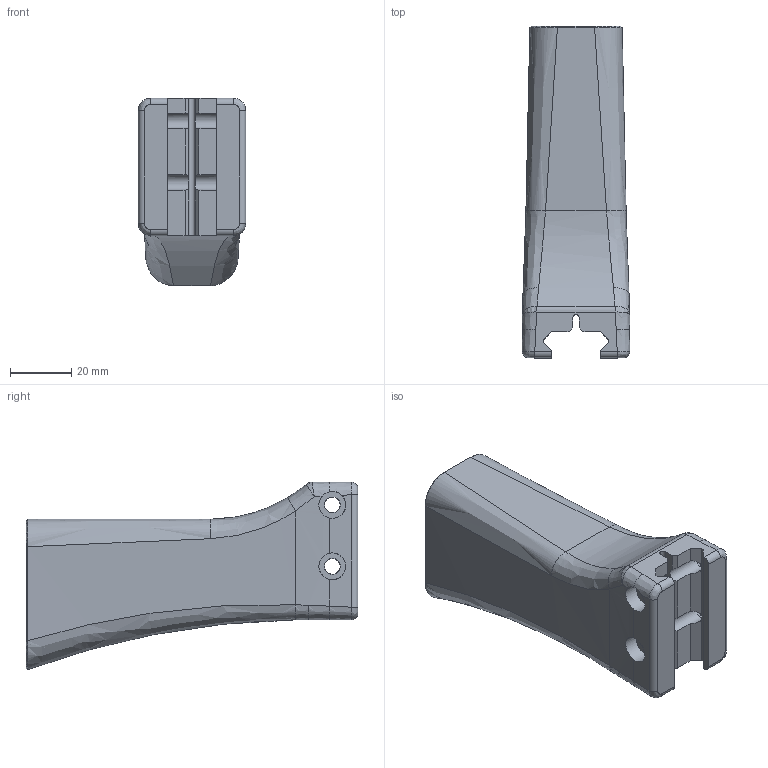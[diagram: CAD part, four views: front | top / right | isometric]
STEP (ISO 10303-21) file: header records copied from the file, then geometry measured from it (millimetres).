
FILE_DESCRIPTION(/* description */ (''),/* implementation_level */ '2;1');
FILE_NAME(/* name */ 'Picatinny Mount.step',/* time_stamp */ '2021-07-28T09:04:42-04:00',/* author */ (''),/* organization */ (''),/* preprocessor_version */ 'ST-DEVELOPER v18.1',/* originating_system */ 'Autodesk Translation Framework v10.9.0.1377',/* authorisation */ '');
FILE_SCHEMA (('AUTOMOTIVE_DESIGN { 1 0 10303 214 3 1 1 }'));
Length unit declared in the file: millimetre
Products named in the file (1): Picatinny Mount
Bounding box: 35 x 108.01 x 61.04 mm (x, y, z)
Volume: 123058.9 mm3; surface area: 21831.8 mm2
Topology: 1 solids, 1 shells, 133 faces, 347 edges, 217 vertices
Faces by surface type: plane 61, bspline 38, cylinder 27, cone 7
Full cylindrical faces by diameter (mm): 5.1 x4, 6.7 x7, 8.75 x2
Entity records: 5129 total; most frequent: CARTESIAN_POINT 2070, ORIENTED_EDGE 690, DIRECTION 521, EDGE_CURVE 345, VERTEX_POINT 217, AXIS2_PLACEMENT_3D 178, LINE 165, VECTOR 165
